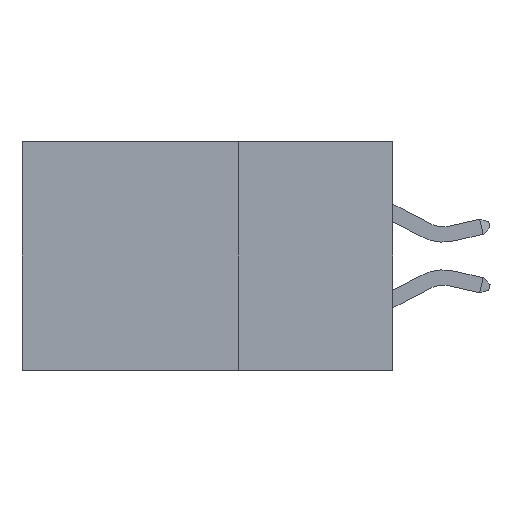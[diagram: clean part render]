
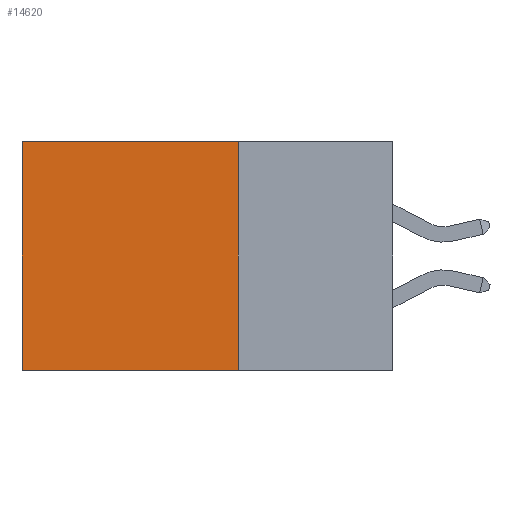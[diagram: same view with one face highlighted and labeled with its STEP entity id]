
A CAD part, left-side view. The second image highlights one B-rep face of the part: STEP entity #14620.
In plain terms, the highlighted planar face has unit normal (-1, 0, 0).
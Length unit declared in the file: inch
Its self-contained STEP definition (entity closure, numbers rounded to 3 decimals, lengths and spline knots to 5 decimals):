
#16 = FACE_OUTER_BOUND ( 'NONE', #6573, .T. ) ;
#156 = ORIENTED_EDGE ( 'NONE', *, *, #2802, .T. ) ;
#1217 = VECTOR ( 'NONE', #11894, 39.37008 ) ;
#1288 = AXIS2_PLACEMENT_3D ( 'NONE', #7724, #4231, #17820 ) ;
#1838 = LINE ( 'NONE', #4179, #1217 ) ;
#2693 = EDGE_CURVE ( 'NONE', #19887, #23685, #1838, .T. ) ;
#2802 = EDGE_CURVE ( 'NONE', #20409, #23685, #13121, .T. ) ;
#3760 = EDGE_CURVE ( 'NONE', #5395, #20409, #11852, .T. ) ;
#4179 = CARTESIAN_POINT ( 'NONE',  ( 0.2875, 0.25, -0.37 ) ) ;
#4231 = DIRECTION ( 'NONE',  ( 1., 0., 0. ) ) ;
#5395 = VERTEX_POINT ( 'NONE', #7402 ) ;
#6573 = EDGE_LOOP ( 'NONE', ( #156, #21207, #14328, #12852 ) ) ;
#7143 = CARTESIAN_POINT ( 'NONE',  ( 0.2875, 0.25, -0.37 ) ) ;
#7402 = CARTESIAN_POINT ( 'NONE',  ( 0.2875, 0.25, 0. ) ) ;
#7634 = LINE ( 'NONE', #25235, #23754 ) ;
#7724 = CARTESIAN_POINT ( 'NONE',  ( 0.2875, 0.25, 0. ) ) ;
#11852 = LINE ( 'NONE', #15945, #20986 ) ;
#11894 = DIRECTION ( 'NONE',  ( 0., 1., 0. ) ) ;
#12852 = ORIENTED_EDGE ( 'NONE', *, *, #3760, .T. ) ;
#13121 = LINE ( 'NONE', #22532, #24091 ) ;
#14328 = ORIENTED_EDGE ( 'NONE', *, *, #16426, .F. ) ;
#14620 = ADVANCED_FACE ( 'NONE', ( #16 ), #17393, .F. ) ;
#15945 = CARTESIAN_POINT ( 'NONE',  ( 0.2875, 0.25, 0. ) ) ;
#16426 = EDGE_CURVE ( 'NONE', #5395, #19887, #7634, .T. ) ;
#17393 = PLANE ( 'NONE',  #1288 ) ;
#17820 = DIRECTION ( 'NONE',  ( 0., 0., -1. ) ) ;
#18067 = DIRECTION ( 'NONE',  ( 0., 1., 0. ) ) ;
#19887 = VERTEX_POINT ( 'NONE', #7143 ) ;
#20409 = VERTEX_POINT ( 'NONE', #25153 ) ;
#20986 = VECTOR ( 'NONE', #18067, 39.37008 ) ;
#21207 = ORIENTED_EDGE ( 'NONE', *, *, #2693, .F. ) ;
#21468 = DIRECTION ( 'NONE',  ( 0., 0., -1. ) ) ;
#22532 = CARTESIAN_POINT ( 'NONE',  ( 0.2875, 0.6, 0. ) ) ;
#23685 = VERTEX_POINT ( 'NONE', #23838 ) ;
#23754 = VECTOR ( 'NONE', #21468, 39.37008 ) ;
#23838 = CARTESIAN_POINT ( 'NONE',  ( 0.2875, 0.6, -0.37 ) ) ;
#24091 = VECTOR ( 'NONE', #24670, 39.37008 ) ;
#24670 = DIRECTION ( 'NONE',  ( 0., 0., -1. ) ) ;
#25153 = CARTESIAN_POINT ( 'NONE',  ( 0.2875, 0.6, 0. ) ) ;
#25235 = CARTESIAN_POINT ( 'NONE',  ( 0.2875, 0.25, 0. ) ) ;
